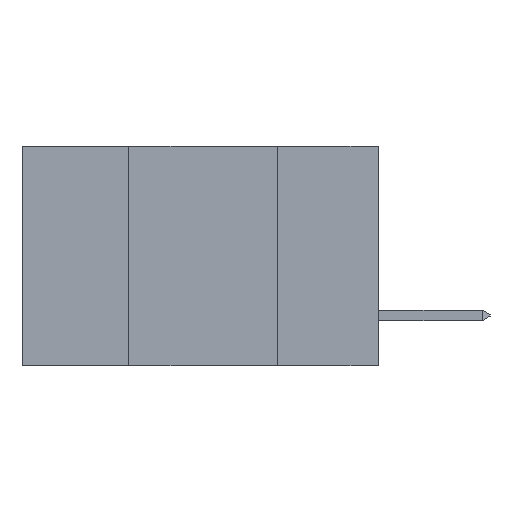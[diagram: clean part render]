
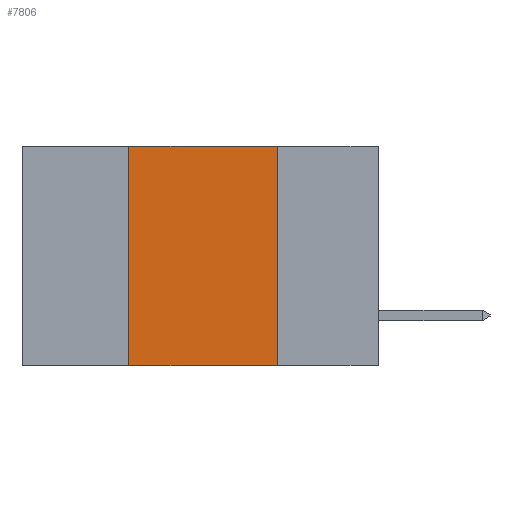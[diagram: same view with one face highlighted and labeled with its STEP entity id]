
A CAD part, left-side view. The second image highlights one B-rep face of the part: STEP entity #7806.
In plain terms, the highlighted planar face has unit normal (-1, 0, 0).
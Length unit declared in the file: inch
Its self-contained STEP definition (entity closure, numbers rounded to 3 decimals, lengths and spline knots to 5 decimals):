
#683 = CARTESIAN_POINT ( 'NONE',  ( 0., 0.6, -0.37 ) ) ;
#1227 = ORIENTED_EDGE ( 'NONE', *, *, #13348, .F. ) ;
#1260 = PLANE ( 'NONE',  #3564 ) ;
#1717 = VERTEX_POINT ( 'NONE', #2419 ) ;
#2419 = CARTESIAN_POINT ( 'NONE',  ( 0., 0.17, 0. ) ) ;
#2461 = CARTESIAN_POINT ( 'NONE',  ( 0., 0.6, 0. ) ) ;
#2516 = DIRECTION ( 'NONE',  ( 0., 0., -1. ) ) ;
#2821 = LINE ( 'NONE', #13831, #12063 ) ;
#3061 = EDGE_LOOP ( 'NONE', ( #1227, #3176, #8587, #7292 ) ) ;
#3132 = EDGE_CURVE ( 'NONE', #11721, #1717, #2821, .T. ) ;
#3176 = ORIENTED_EDGE ( 'NONE', *, *, #3132, .F. ) ;
#3484 = LINE ( 'NONE', #10852, #9611 ) ;
#3564 = AXIS2_PLACEMENT_3D ( 'NONE', #2461, #9832, #2516 ) ;
#3801 = CARTESIAN_POINT ( 'NONE',  ( 0., 0.42, 0. ) ) ;
#4472 = EDGE_CURVE ( 'NONE', #11533, #11721, #3484, .T. ) ;
#4929 = VECTOR ( 'NONE', #10464, 39.37008 ) ;
#5199 = LINE ( 'NONE', #7321, #8834 ) ;
#7292 = ORIENTED_EDGE ( 'NONE', *, *, #7509, .T. ) ;
#7321 = CARTESIAN_POINT ( 'NONE',  ( 0., 0.17, 0. ) ) ;
#7509 = EDGE_CURVE ( 'NONE', #11533, #10649, #11676, .T. ) ;
#7806 = ADVANCED_FACE ( 'NONE', ( #13442 ), #1260, .F. ) ;
#8587 = ORIENTED_EDGE ( 'NONE', *, *, #4472, .F. ) ;
#8834 = VECTOR ( 'NONE', #15400, 39.37008 ) ;
#9611 = VECTOR ( 'NONE', #10718, 39.37008 ) ;
#9832 = DIRECTION ( 'NONE',  ( 1., 0., 0. ) ) ;
#10464 = DIRECTION ( 'NONE',  ( 0., -1., 0. ) ) ;
#10649 = VERTEX_POINT ( 'NONE', #13360 ) ;
#10718 = DIRECTION ( 'NONE',  ( 0., 0., 1. ) ) ;
#10739 = CARTESIAN_POINT ( 'NONE',  ( 0., 0.42, -0.37 ) ) ;
#10852 = CARTESIAN_POINT ( 'NONE',  ( 0., 0.42, 0. ) ) ;
#11533 = VERTEX_POINT ( 'NONE', #10739 ) ;
#11676 = LINE ( 'NONE', #683, #4929 ) ;
#11721 = VERTEX_POINT ( 'NONE', #3801 ) ;
#12063 = VECTOR ( 'NONE', #13992, 39.37008 ) ;
#13348 = EDGE_CURVE ( 'NONE', #1717, #10649, #5199, .T. ) ;
#13360 = CARTESIAN_POINT ( 'NONE',  ( 0., 0.17, -0.37 ) ) ;
#13442 = FACE_OUTER_BOUND ( 'NONE', #3061, .T. ) ;
#13831 = CARTESIAN_POINT ( 'NONE',  ( 0., 0.6, 0. ) ) ;
#13992 = DIRECTION ( 'NONE',  ( 0., -1., 0. ) ) ;
#15400 = DIRECTION ( 'NONE',  ( 0., 0., -1. ) ) ;
